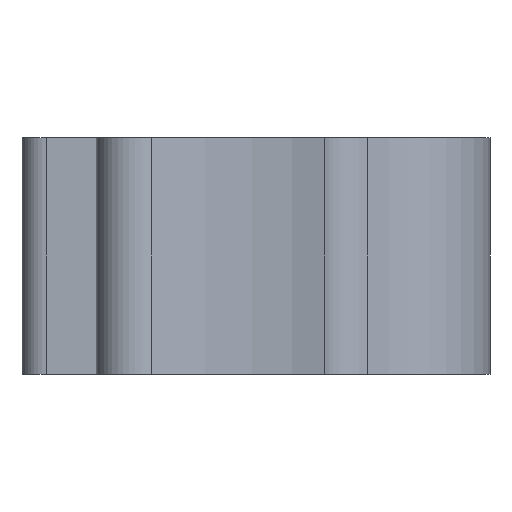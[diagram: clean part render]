
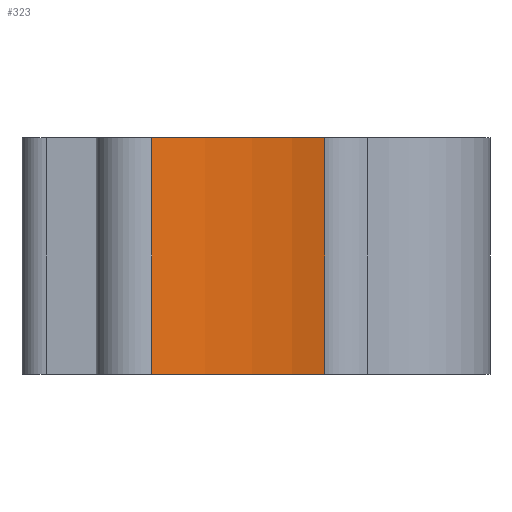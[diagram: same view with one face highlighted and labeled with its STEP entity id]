
A CAD part, front view. The second image highlights one B-rep face of the part: STEP entity #323.
In plain terms, the highlighted cylindrical face has radius 19.419 mm (diameter 38.838 mm), a partial arc.
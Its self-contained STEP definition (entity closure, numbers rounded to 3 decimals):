
#18 = EDGE_CURVE ( 'NONE', #513, #558, #543, .T. ) ;
#49 = DIRECTION ( 'NONE',  ( 0., 0., 1. ) ) ;
#59 = CARTESIAN_POINT ( 'NONE',  ( 82.849, -3.115, 8.85 ) ) ;
#78 = FACE_OUTER_BOUND ( 'NONE', #774, .T. ) ;
#175 = VECTOR ( 'NONE', #49, 1000. ) ;
#185 = CARTESIAN_POINT ( 'NONE',  ( 89.977, 5.009, -0.9 ) ) ;
#222 = LINE ( 'NONE', #185, #175 ) ;
#249 = DIRECTION ( 'NONE',  ( 1., 0., 0. ) ) ;
#262 = AXIS2_PLACEMENT_3D ( 'NONE', #412, #861, #482 ) ;
#267 = CIRCLE ( 'NONE', #262, 19.419 ) ;
#291 = EDGE_CURVE ( 'NONE', #704, #558, #222, .T. ) ;
#314 = AXIS2_PLACEMENT_3D ( 'NONE', #466, #598, #461 ) ;
#323 = ADVANCED_FACE ( 'NONE', ( #78 ), #778, .T. ) ;
#398 = CARTESIAN_POINT ( 'NONE',  ( 82.849, -3.115, -0.9 ) ) ;
#412 = CARTESIAN_POINT ( 'NONE',  ( 72.393, 13.249, -0.9 ) ) ;
#421 = CARTESIAN_POINT ( 'NONE',  ( 72.393, 13.249, -0.9 ) ) ;
#429 = ORIENTED_EDGE ( 'NONE', *, *, #18, .F. ) ;
#461 = DIRECTION ( 'NONE',  ( 1., 0., 0. ) ) ;
#462 = ORIENTED_EDGE ( 'NONE', *, *, #580, .T. ) ;
#463 = ORIENTED_EDGE ( 'NONE', *, *, #695, .T. ) ;
#466 = CARTESIAN_POINT ( 'NONE',  ( 72.393, 13.249, 8.85 ) ) ;
#482 = DIRECTION ( 'NONE',  ( 1., 0., 0. ) ) ;
#513 = VERTEX_POINT ( 'NONE', #59 ) ;
#522 = VERTEX_POINT ( 'NONE', #398 ) ;
#543 = CIRCLE ( 'NONE', #314, 19.419 ) ;
#545 = DIRECTION ( 'NONE',  ( 0., 0., 1. ) ) ;
#558 = VERTEX_POINT ( 'NONE', #800 ) ;
#580 = EDGE_CURVE ( 'NONE', #522, #704, #267, .T. ) ;
#598 = DIRECTION ( 'NONE',  ( 0., 0., 1. ) ) ;
#628 = CARTESIAN_POINT ( 'NONE',  ( 82.849, -3.115, -0.9 ) ) ;
#630 = DIRECTION ( 'NONE',  ( 0., 0., -1. ) ) ;
#668 = ORIENTED_EDGE ( 'NONE', *, *, #291, .T. ) ;
#669 = VECTOR ( 'NONE', #630, 1000. ) ;
#694 = CARTESIAN_POINT ( 'NONE',  ( 89.977, 5.009, -0.9 ) ) ;
#695 = EDGE_CURVE ( 'NONE', #513, #522, #838, .T. ) ;
#704 = VERTEX_POINT ( 'NONE', #694 ) ;
#774 = EDGE_LOOP ( 'NONE', ( #429, #463, #462, #668 ) ) ;
#778 = CYLINDRICAL_SURFACE ( 'NONE', #839, 19.419 ) ;
#800 = CARTESIAN_POINT ( 'NONE',  ( 89.977, 5.009, 8.85 ) ) ;
#838 = LINE ( 'NONE', #628, #669 ) ;
#839 = AXIS2_PLACEMENT_3D ( 'NONE', #421, #545, #249 ) ;
#861 = DIRECTION ( 'NONE',  ( 0., 0., 1. ) ) ;
